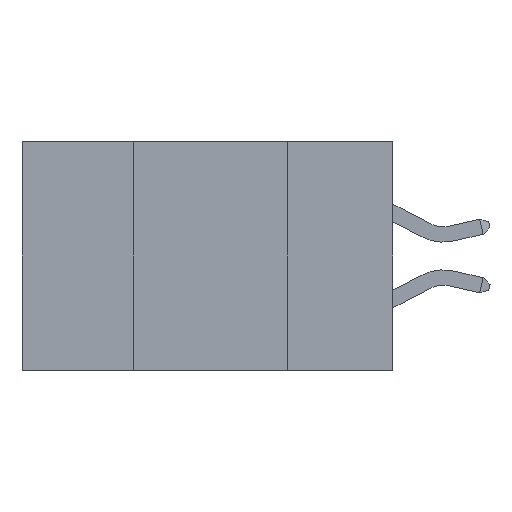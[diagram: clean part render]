
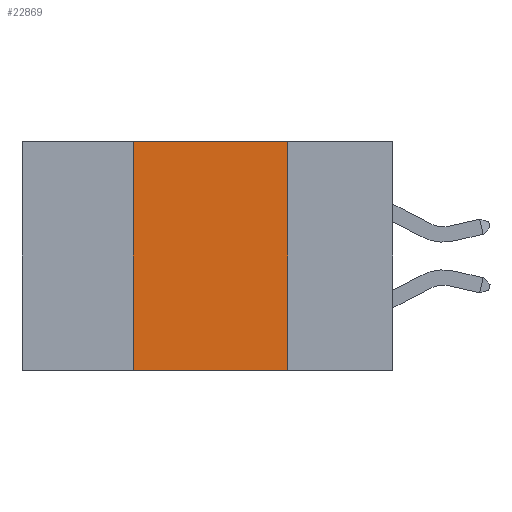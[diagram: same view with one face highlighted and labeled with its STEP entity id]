
A CAD part, left-side view. The second image highlights one B-rep face of the part: STEP entity #22869.
In plain terms, the highlighted planar face has unit normal (-1, 0, 0).
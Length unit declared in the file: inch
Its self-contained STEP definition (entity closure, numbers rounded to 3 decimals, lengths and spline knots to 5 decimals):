
#717 = VECTOR ( 'NONE', #24783, 39.37008 ) ;
#2304 = CARTESIAN_POINT ( 'NONE',  ( 0., 0.42, 0. ) ) ;
#3027 = LINE ( 'NONE', #15958, #717 ) ;
#3460 = VERTEX_POINT ( 'NONE', #26158 ) ;
#4814 = VERTEX_POINT ( 'NONE', #15930 ) ;
#6425 = EDGE_LOOP ( 'NONE', ( #10899, #21971, #26468, #16160 ) ) ;
#7832 = CARTESIAN_POINT ( 'NONE',  ( 0., 0.42, 0. ) ) ;
#8181 = DIRECTION ( 'NONE',  ( 0., -1., 0. ) ) ;
#8380 = LINE ( 'NONE', #2304, #13315 ) ;
#9056 = EDGE_CURVE ( 'NONE', #24703, #4814, #3027, .T. ) ;
#9247 = FACE_OUTER_BOUND ( 'NONE', #6425, .T. ) ;
#10856 = DIRECTION ( 'NONE',  ( 0., 0., 1. ) ) ;
#10899 = ORIENTED_EDGE ( 'NONE', *, *, #9056, .F. ) ;
#11853 = LINE ( 'NONE', #17595, #27449 ) ;
#11949 = CARTESIAN_POINT ( 'NONE',  ( 0., 0.6, 0. ) ) ;
#13315 = VECTOR ( 'NONE', #10856, 39.37008 ) ;
#13579 = VECTOR ( 'NONE', #8181, 39.37008 ) ;
#13892 = PLANE ( 'NONE',  #22190 ) ;
#13967 = EDGE_CURVE ( 'NONE', #23601, #24703, #25865, .T. ) ;
#15506 = EDGE_CURVE ( 'NONE', #3460, #4814, #11853, .T. ) ;
#15930 = CARTESIAN_POINT ( 'NONE',  ( 0., 0.17, -0.37 ) ) ;
#15958 = CARTESIAN_POINT ( 'NONE',  ( 0., 0.17, 0. ) ) ;
#16160 = ORIENTED_EDGE ( 'NONE', *, *, #15506, .T. ) ;
#16292 = DIRECTION ( 'NONE',  ( 1., 0., 0. ) ) ;
#17426 = DIRECTION ( 'NONE',  ( 0., -1., 0. ) ) ;
#17595 = CARTESIAN_POINT ( 'NONE',  ( 0., 0.6, -0.37 ) ) ;
#18523 = CARTESIAN_POINT ( 'NONE',  ( 0., 0.6, 0. ) ) ;
#20368 = DIRECTION ( 'NONE',  ( 0., 0., -1. ) ) ;
#20419 = CARTESIAN_POINT ( 'NONE',  ( 0., 0.17, 0. ) ) ;
#21038 = EDGE_CURVE ( 'NONE', #3460, #23601, #8380, .T. ) ;
#21971 = ORIENTED_EDGE ( 'NONE', *, *, #13967, .F. ) ;
#22190 = AXIS2_PLACEMENT_3D ( 'NONE', #11949, #16292, #20368 ) ;
#22869 = ADVANCED_FACE ( 'NONE', ( #9247 ), #13892, .F. ) ;
#23601 = VERTEX_POINT ( 'NONE', #7832 ) ;
#24703 = VERTEX_POINT ( 'NONE', #20419 ) ;
#24783 = DIRECTION ( 'NONE',  ( 0., 0., -1. ) ) ;
#25865 = LINE ( 'NONE', #18523, #13579 ) ;
#26158 = CARTESIAN_POINT ( 'NONE',  ( 0., 0.42, -0.37 ) ) ;
#26468 = ORIENTED_EDGE ( 'NONE', *, *, #21038, .F. ) ;
#27449 = VECTOR ( 'NONE', #17426, 39.37008 ) ;
